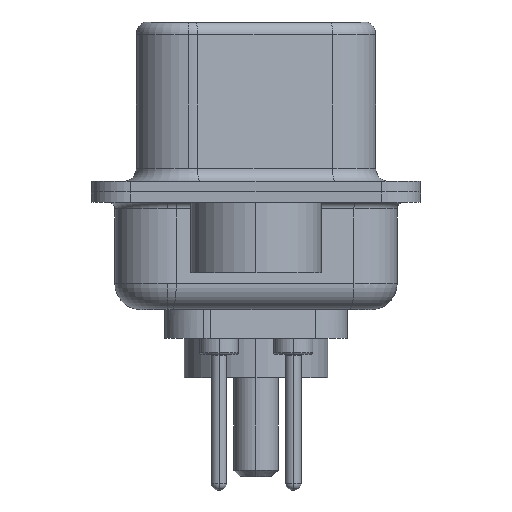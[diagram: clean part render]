
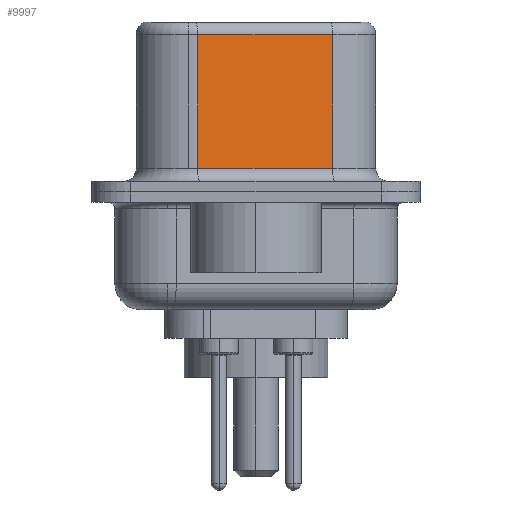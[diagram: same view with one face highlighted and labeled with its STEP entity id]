
A CAD part, left-side view. The second image highlights one B-rep face of the part: STEP entity #9997.
In plain terms, the highlighted planar face has unit normal (-0.985, -0.174, 0).
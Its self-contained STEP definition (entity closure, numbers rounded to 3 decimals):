
#1311 = ORIENTED_EDGE ( 'NONE', *, *, #11864, .T. ) ;
#1687 = CARTESIAN_POINT ( 'NONE',  ( 4.58, -2.927, 0.9 ) ) ;
#1936 = VERTEX_POINT ( 'NONE', #12504 ) ;
#2097 = VECTOR ( 'NONE', #13837, 1000. ) ;
#2558 = LINE ( 'NONE', #3988, #4746 ) ;
#2862 = CARTESIAN_POINT ( 'NONE',  ( 3.67, 2.233, 6.52 ) ) ;
#3177 = CARTESIAN_POINT ( 'NONE',  ( 4.58, -2.927, 0.9 ) ) ;
#3320 = DIRECTION ( 'NONE',  ( 0.985, 0.174, 0. ) ) ;
#3609 = EDGE_CURVE ( 'NONE', #13246, #3827, #5362, .T. ) ;
#3827 = VERTEX_POINT ( 'NONE', #6939 ) ;
#3988 = CARTESIAN_POINT ( 'NONE',  ( 4.58, -2.927, 6.02 ) ) ;
#4746 = VECTOR ( 'NONE', #13792, 1000. ) ;
#5362 = LINE ( 'NONE', #2862, #2097 ) ;
#5734 = EDGE_CURVE ( 'NONE', #1936, #13246, #2558, .T. ) ;
#5984 = ORIENTED_EDGE ( 'NONE', *, *, #5734, .T. ) ;
#6410 = CARTESIAN_POINT ( 'NONE',  ( 4.58, -2.927, 6.52 ) ) ;
#6566 = VECTOR ( 'NONE', #13827, 1000. ) ;
#6607 = PLANE ( 'NONE',  #12398 ) ;
#6939 = CARTESIAN_POINT ( 'NONE',  ( 3.67, 2.233, 0.9 ) ) ;
#7965 = FACE_OUTER_BOUND ( 'NONE', #13542, .T. ) ;
#9854 = LINE ( 'NONE', #6410, #12818 ) ;
#9997 = ADVANCED_FACE ( 'NONE', ( #7965 ), #6607, .F. ) ;
#10896 = DIRECTION ( 'NONE',  ( -0.174, 0.985, 0. ) ) ;
#11476 = VERTEX_POINT ( 'NONE', #1687 ) ;
#11529 = ORIENTED_EDGE ( 'NONE', *, *, #3609, .T. ) ;
#11784 = EDGE_CURVE ( 'NONE', #1936, #11476, #9854, .T. ) ;
#11860 = LINE ( 'NONE', #3177, #6566 ) ;
#11864 = EDGE_CURVE ( 'NONE', #3827, #11476, #11860, .T. ) ;
#12398 = AXIS2_PLACEMENT_3D ( 'NONE', #12892, #3320, #10896 ) ;
#12504 = CARTESIAN_POINT ( 'NONE',  ( 4.58, -2.927, 6.02 ) ) ;
#12818 = VECTOR ( 'NONE', #13776, 1000. ) ;
#12892 = CARTESIAN_POINT ( 'NONE',  ( 4.58, -2.927, 6.52 ) ) ;
#13246 = VERTEX_POINT ( 'NONE', #13979 ) ;
#13542 = EDGE_LOOP ( 'NONE', ( #14007, #5984, #11529, #1311 ) ) ;
#13776 = DIRECTION ( 'NONE',  ( 0., 0., -1. ) ) ;
#13792 = DIRECTION ( 'NONE',  ( -0.174, 0.985, 0. ) ) ;
#13827 = DIRECTION ( 'NONE',  ( 0.174, -0.985, 0. ) ) ;
#13837 = DIRECTION ( 'NONE',  ( 0., 0., -1. ) ) ;
#13979 = CARTESIAN_POINT ( 'NONE',  ( 3.67, 2.233, 6.02 ) ) ;
#14007 = ORIENTED_EDGE ( 'NONE', *, *, #11784, .F. ) ;
